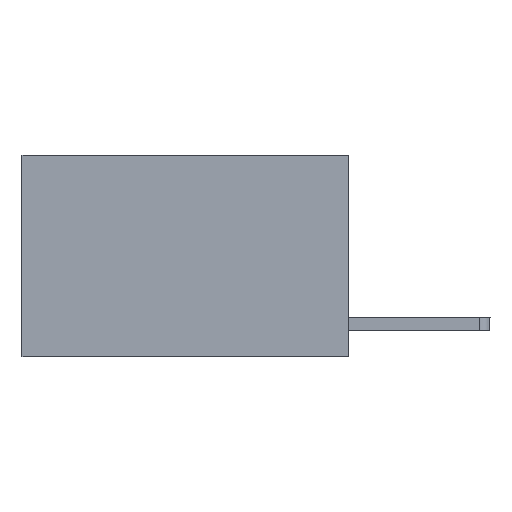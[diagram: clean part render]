
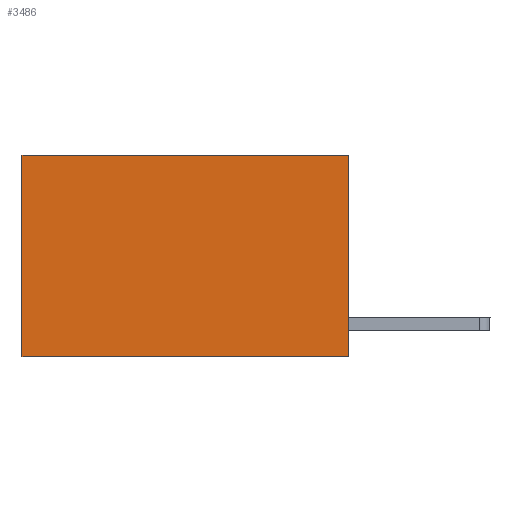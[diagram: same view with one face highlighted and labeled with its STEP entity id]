
A CAD part, left-side view. The second image highlights one B-rep face of the part: STEP entity #3486.
In plain terms, the highlighted planar face has unit normal (-1, 0, 0).
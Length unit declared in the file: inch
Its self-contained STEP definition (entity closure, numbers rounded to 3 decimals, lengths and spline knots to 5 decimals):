
#524 = VERTEX_POINT ( 'NONE', #2243 ) ;
#855 = CARTESIAN_POINT ( 'NONE',  ( 0.2625, 0., 0. ) ) ;
#1114 = CARTESIAN_POINT ( 'NONE',  ( 0.2625, 0., 0. ) ) ;
#1266 = VERTEX_POINT ( 'NONE', #2795 ) ;
#1559 = VECTOR ( 'NONE', #12483, 39.37008 ) ;
#2243 = CARTESIAN_POINT ( 'NONE',  ( 0.2625, 0., 0. ) ) ;
#2467 = ORIENTED_EDGE ( 'NONE', *, *, #10072, .T. ) ;
#2474 = VECTOR ( 'NONE', #6519, 39.37008 ) ;
#2584 = LINE ( 'NONE', #3546, #1559 ) ;
#2622 = LINE ( 'NONE', #7277, #2474 ) ;
#2795 = CARTESIAN_POINT ( 'NONE',  ( 0.2625, 0.6, 0. ) ) ;
#2854 = AXIS2_PLACEMENT_3D ( 'NONE', #1114, #3090, #6025 ) ;
#3090 = DIRECTION ( 'NONE',  ( 1., 0., 0. ) ) ;
#3486 = ADVANCED_FACE ( 'NONE', ( #8881 ), #5189, .F. ) ;
#3546 = CARTESIAN_POINT ( 'NONE',  ( 0.2625, 0., 0. ) ) ;
#4299 = EDGE_CURVE ( 'NONE', #524, #1266, #2584, .T. ) ;
#4634 = CARTESIAN_POINT ( 'NONE',  ( 0.2625, 0., -0.37 ) ) ;
#4739 = DIRECTION ( 'NONE',  ( 0., 0., -1. ) ) ;
#4979 = DIRECTION ( 'NONE',  ( 0., 1., 0. ) ) ;
#5189 = PLANE ( 'NONE',  #2854 ) ;
#5556 = LINE ( 'NONE', #855, #8982 ) ;
#5740 = VERTEX_POINT ( 'NONE', #4634 ) ;
#6025 = DIRECTION ( 'NONE',  ( 0., 0., -1. ) ) ;
#6519 = DIRECTION ( 'NONE',  ( 0., 0., -1. ) ) ;
#7277 = CARTESIAN_POINT ( 'NONE',  ( 0.2625, 0.6, 0. ) ) ;
#7867 = EDGE_LOOP ( 'NONE', ( #2467, #11635, #11298, #11397 ) ) ;
#8242 = EDGE_CURVE ( 'NONE', #5740, #8400, #10783, .T. ) ;
#8400 = VERTEX_POINT ( 'NONE', #8845 ) ;
#8845 = CARTESIAN_POINT ( 'NONE',  ( 0.2625, 0.6, -0.37 ) ) ;
#8881 = FACE_OUTER_BOUND ( 'NONE', #7867, .T. ) ;
#8982 = VECTOR ( 'NONE', #4739, 39.37008 ) ;
#9738 = VECTOR ( 'NONE', #4979, 39.37008 ) ;
#10072 = EDGE_CURVE ( 'NONE', #1266, #8400, #2622, .T. ) ;
#10136 = EDGE_CURVE ( 'NONE', #524, #5740, #5556, .T. ) ;
#10659 = CARTESIAN_POINT ( 'NONE',  ( 0.2625, 0., -0.37 ) ) ;
#10783 = LINE ( 'NONE', #10659, #9738 ) ;
#11298 = ORIENTED_EDGE ( 'NONE', *, *, #10136, .F. ) ;
#11397 = ORIENTED_EDGE ( 'NONE', *, *, #4299, .T. ) ;
#11635 = ORIENTED_EDGE ( 'NONE', *, *, #8242, .F. ) ;
#12483 = DIRECTION ( 'NONE',  ( 0., 1., 0. ) ) ;
